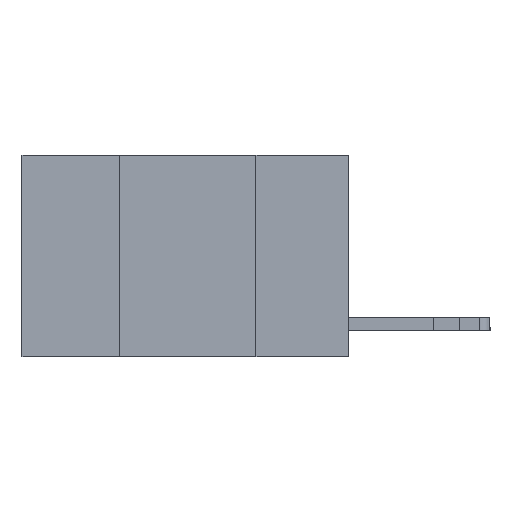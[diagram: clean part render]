
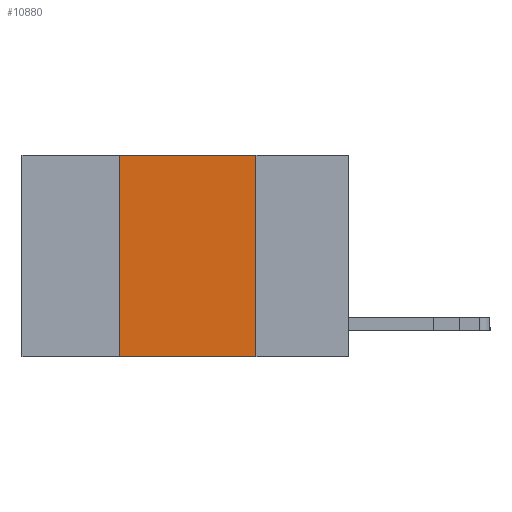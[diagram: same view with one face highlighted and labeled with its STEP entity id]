
A CAD part, left-side view. The second image highlights one B-rep face of the part: STEP entity #10880.
In plain terms, the highlighted planar face has unit normal (-1, 0, 0).
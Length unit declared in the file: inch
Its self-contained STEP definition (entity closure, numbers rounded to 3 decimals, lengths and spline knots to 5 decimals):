
#652 = EDGE_CURVE ( 'NONE', #794, #13217, #6915, .T. ) ;
#794 = VERTEX_POINT ( 'NONE', #16110 ) ;
#1146 = EDGE_CURVE ( 'NONE', #13217, #15101, #3259, .T. ) ;
#1334 = PLANE ( 'NONE',  #13920 ) ;
#1360 = CARTESIAN_POINT ( 'NONE',  ( 0., 0.17, -0.37 ) ) ;
#2928 = DIRECTION ( 'NONE',  ( 0., -1., 0. ) ) ;
#3259 = LINE ( 'NONE', #4678, #9239 ) ;
#3578 = LINE ( 'NONE', #8614, #12886 ) ;
#3820 = EDGE_CURVE ( 'NONE', #5919, #15101, #10501, .T. ) ;
#4678 = CARTESIAN_POINT ( 'NONE',  ( 0., 0.17, 0. ) ) ;
#4777 = EDGE_LOOP ( 'NONE', ( #12105, #5138, #14306, #7793 ) ) ;
#5138 = ORIENTED_EDGE ( 'NONE', *, *, #652, .F. ) ;
#5919 = VERTEX_POINT ( 'NONE', #8791 ) ;
#6359 = DIRECTION ( 'NONE',  ( 1., 0., 0. ) ) ;
#6915 = LINE ( 'NONE', #14513, #14050 ) ;
#7793 = ORIENTED_EDGE ( 'NONE', *, *, #3820, .T. ) ;
#7879 = CARTESIAN_POINT ( 'NONE',  ( 0., 0.6, 0. ) ) ;
#8614 = CARTESIAN_POINT ( 'NONE',  ( 0., 0.42, 0. ) ) ;
#8791 = CARTESIAN_POINT ( 'NONE',  ( 0., 0.42, -0.37 ) ) ;
#9223 = CARTESIAN_POINT ( 'NONE',  ( 0., 0.6, -0.37 ) ) ;
#9239 = VECTOR ( 'NONE', #14713, 39.37008 ) ;
#10501 = LINE ( 'NONE', #9223, #15848 ) ;
#10880 = ADVANCED_FACE ( 'NONE', ( #15548 ), #1334, .F. ) ;
#10969 = DIRECTION ( 'NONE',  ( 0., -1., 0. ) ) ;
#11345 = DIRECTION ( 'NONE',  ( 0., 0., -1. ) ) ;
#12105 = ORIENTED_EDGE ( 'NONE', *, *, #1146, .F. ) ;
#12886 = VECTOR ( 'NONE', #15347, 39.37008 ) ;
#13161 = CARTESIAN_POINT ( 'NONE',  ( 0., 0.17, 0. ) ) ;
#13217 = VERTEX_POINT ( 'NONE', #13161 ) ;
#13920 = AXIS2_PLACEMENT_3D ( 'NONE', #7879, #6359, #11345 ) ;
#14050 = VECTOR ( 'NONE', #10969, 39.37008 ) ;
#14306 = ORIENTED_EDGE ( 'NONE', *, *, #14440, .F. ) ;
#14440 = EDGE_CURVE ( 'NONE', #5919, #794, #3578, .T. ) ;
#14513 = CARTESIAN_POINT ( 'NONE',  ( 0., 0.6, 0. ) ) ;
#14713 = DIRECTION ( 'NONE',  ( 0., 0., -1. ) ) ;
#15101 = VERTEX_POINT ( 'NONE', #1360 ) ;
#15347 = DIRECTION ( 'NONE',  ( 0., 0., 1. ) ) ;
#15548 = FACE_OUTER_BOUND ( 'NONE', #4777, .T. ) ;
#15848 = VECTOR ( 'NONE', #2928, 39.37008 ) ;
#16110 = CARTESIAN_POINT ( 'NONE',  ( 0., 0.42, 0. ) ) ;
